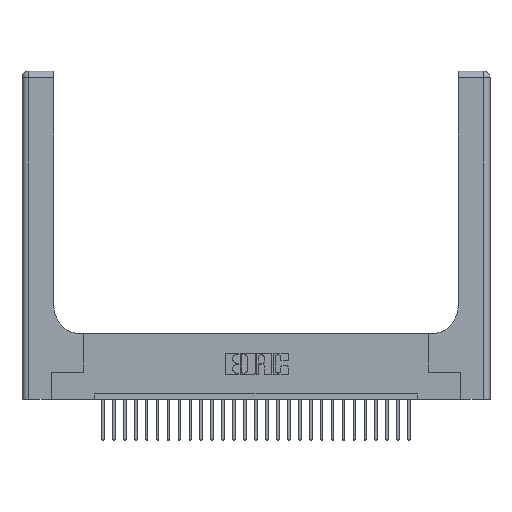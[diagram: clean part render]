
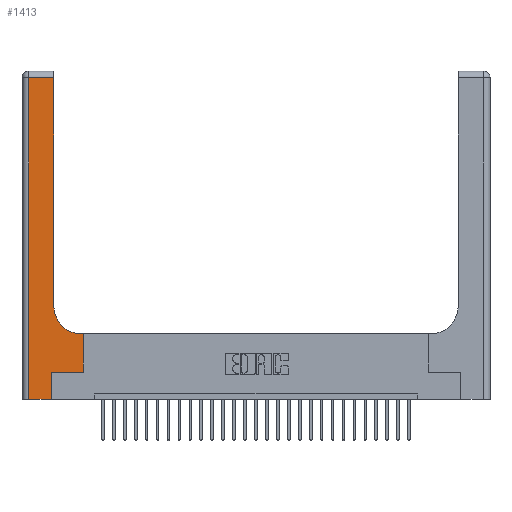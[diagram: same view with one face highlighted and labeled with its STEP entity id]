
A CAD part, top view. The second image highlights one B-rep face of the part: STEP entity #1413.
In plain terms, the highlighted planar face has unit normal (0, 0, 1).
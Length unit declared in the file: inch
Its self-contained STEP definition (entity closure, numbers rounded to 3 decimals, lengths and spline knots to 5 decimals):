
#1041 = DIRECTION ( 'NONE',  ( 0., 0., -1. ) ) ;
#1285 = LINE ( 'NONE', #2177, #5448 ) ;
#1399 = ORIENTED_EDGE ( 'NONE', *, *, #24659, .T. ) ;
#1413 = ADVANCED_FACE ( 'NONE', ( #11473 ), #11850, .F. ) ;
#1582 = DIRECTION ( 'NONE',  ( -1., 0., 0. ) ) ;
#2157 = DIRECTION ( 'NONE',  ( 0., 1., 0. ) ) ;
#2177 = CARTESIAN_POINT ( 'NONE',  ( 0., 2.94, 0.37 ) ) ;
#2269 = CARTESIAN_POINT ( 'NONE',  ( 0.2915, 2.94, 0.37 ) ) ;
#2409 = DIRECTION ( 'NONE',  ( 0., 0., -1. ) ) ;
#2618 = VECTOR ( 'NONE', #4669, 39.37008 ) ;
#2791 = VERTEX_POINT ( 'NONE', #10777 ) ;
#2943 = ORIENTED_EDGE ( 'NONE', *, *, #15531, .T. ) ;
#3186 = ORIENTED_EDGE ( 'NONE', *, *, #28336, .T. ) ;
#3301 = DIRECTION ( 'NONE',  ( 0., 1., 0. ) ) ;
#3446 = DIRECTION ( 'NONE',  ( 0., -1., 0. ) ) ;
#3562 = LINE ( 'NONE', #14528, #13965 ) ;
#3568 = ORIENTED_EDGE ( 'NONE', *, *, #21527, .T. ) ;
#3612 = CARTESIAN_POINT ( 'NONE',  ( 0.2915, 0.85, 0.37 ) ) ;
#4049 = EDGE_CURVE ( 'NONE', #25905, #8226, #11655, .T. ) ;
#4669 = DIRECTION ( 'NONE',  ( 0., 1., 0. ) ) ;
#5226 = ORIENTED_EDGE ( 'NONE', *, *, #14242, .T. ) ;
#5299 = VERTEX_POINT ( 'NONE', #6843 ) ;
#5448 = VECTOR ( 'NONE', #17735, 39.37008 ) ;
#6843 = CARTESIAN_POINT ( 'NONE',  ( 0.5585, 0.6, 0.37 ) ) ;
#8205 = VERTEX_POINT ( 'NONE', #28719 ) ;
#8226 = VERTEX_POINT ( 'NONE', #2269 ) ;
#8945 = EDGE_LOOP ( 'NONE', ( #27321, #3186, #2943, #28322, #5226, #17692, #1399, #14271, #3568 ) ) ;
#9003 = CARTESIAN_POINT ( 'NONE',  ( 0.2915, 3., 0.37 ) ) ;
#9854 = DIRECTION ( 'NONE',  ( -1., 0., 0. ) ) ;
#9930 = AXIS2_PLACEMENT_3D ( 'NONE', #13382, #2409, #20267 ) ;
#10163 = CARTESIAN_POINT ( 'NONE',  ( 0.269, 0., 0.37 ) ) ;
#10542 = LINE ( 'NONE', #21708, #28271 ) ;
#10654 = CARTESIAN_POINT ( 'NONE',  ( 0., 0., 0.37 ) ) ;
#10757 = DIRECTION ( 'NONE',  ( 1., 0., 0. ) ) ;
#10777 = CARTESIAN_POINT ( 'NONE',  ( 0.5415, 0.6, 0.37 ) ) ;
#11473 = FACE_OUTER_BOUND ( 'NONE', #8945, .T. ) ;
#11655 = LINE ( 'NONE', #9003, #2618 ) ;
#11850 = PLANE ( 'NONE',  #26556 ) ;
#12148 = CARTESIAN_POINT ( 'NONE',  ( 0., 3., 0.37 ) ) ;
#13293 = VERTEX_POINT ( 'NONE', #23770 ) ;
#13382 = CARTESIAN_POINT ( 'NONE',  ( 0.5415, 0.85, 0.37 ) ) ;
#13636 = LINE ( 'NONE', #17534, #28236 ) ;
#13678 = VERTEX_POINT ( 'NONE', #23549 ) ;
#13965 = VECTOR ( 'NONE', #3446, 39.37008 ) ;
#14242 = EDGE_CURVE ( 'NONE', #18085, #8205, #15487, .T. ) ;
#14271 = ORIENTED_EDGE ( 'NONE', *, *, #24458, .T. ) ;
#14528 = CARTESIAN_POINT ( 'NONE',  ( 0.06, 3., 0.37 ) ) ;
#15487 = LINE ( 'NONE', #16604, #21315 ) ;
#15531 = EDGE_CURVE ( 'NONE', #13678, #25578, #3562, .T. ) ;
#15791 = LINE ( 'NONE', #17308, #26243 ) ;
#16604 = CARTESIAN_POINT ( 'NONE',  ( 0.269, 0., 0.37 ) ) ;
#16605 = CARTESIAN_POINT ( 'NONE',  ( 0.06, 0., 0.37 ) ) ;
#17308 = CARTESIAN_POINT ( 'NONE',  ( 0.269, 0.25, 0.37 ) ) ;
#17534 = CARTESIAN_POINT ( 'NONE',  ( 0.5585, 0.25, 0.37 ) ) ;
#17692 = ORIENTED_EDGE ( 'NONE', *, *, #20072, .T. ) ;
#17735 = DIRECTION ( 'NONE',  ( -1., 0., 0. ) ) ;
#18085 = VERTEX_POINT ( 'NONE', #10163 ) ;
#18296 = VECTOR ( 'NONE', #10757, 39.37008 ) ;
#18453 = EDGE_CURVE ( 'NONE', #25578, #18085, #21095, .T. ) ;
#20072 = EDGE_CURVE ( 'NONE', #8205, #13293, #15791, .T. ) ;
#20267 = DIRECTION ( 'NONE',  ( 1., 0., 0. ) ) ;
#21095 = LINE ( 'NONE', #10654, #18296 ) ;
#21315 = VECTOR ( 'NONE', #3301, 39.37008 ) ;
#21527 = EDGE_CURVE ( 'NONE', #2791, #25905, #26692, .T. ) ;
#21708 = CARTESIAN_POINT ( 'NONE',  ( 0.2915, 0.6, 0.37 ) ) ;
#23549 = CARTESIAN_POINT ( 'NONE',  ( 0.06, 2.94, 0.37 ) ) ;
#23770 = CARTESIAN_POINT ( 'NONE',  ( 0.5585, 0.25, 0.37 ) ) ;
#24458 = EDGE_CURVE ( 'NONE', #5299, #2791, #10542, .T. ) ;
#24465 = DIRECTION ( 'NONE',  ( 1., 0., 0. ) ) ;
#24659 = EDGE_CURVE ( 'NONE', #13293, #5299, #13636, .T. ) ;
#25578 = VERTEX_POINT ( 'NONE', #16605 ) ;
#25905 = VERTEX_POINT ( 'NONE', #3612 ) ;
#26243 = VECTOR ( 'NONE', #24465, 39.37008 ) ;
#26556 = AXIS2_PLACEMENT_3D ( 'NONE', #12148, #1041, #9854 ) ;
#26692 = CIRCLE ( 'NONE', #9930, 0.25 ) ;
#27321 = ORIENTED_EDGE ( 'NONE', *, *, #4049, .T. ) ;
#28236 = VECTOR ( 'NONE', #2157, 39.37008 ) ;
#28271 = VECTOR ( 'NONE', #1582, 39.37008 ) ;
#28322 = ORIENTED_EDGE ( 'NONE', *, *, #18453, .T. ) ;
#28336 = EDGE_CURVE ( 'NONE', #8226, #13678, #1285, .T. ) ;
#28719 = CARTESIAN_POINT ( 'NONE',  ( 0.269, 0.25, 0.37 ) ) ;
